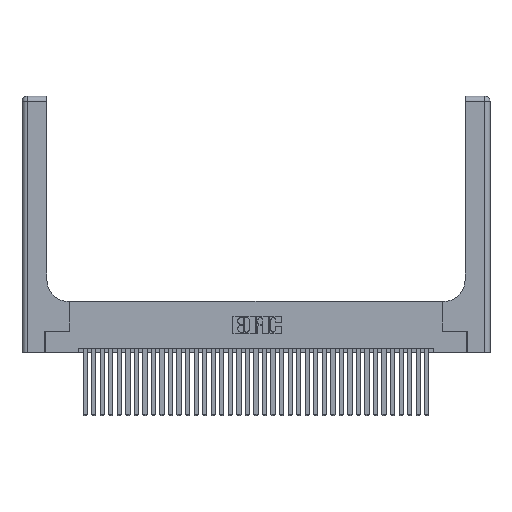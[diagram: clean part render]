
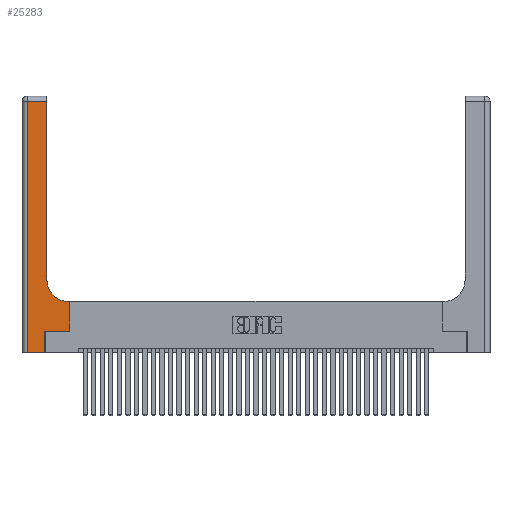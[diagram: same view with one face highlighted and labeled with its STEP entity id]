
A CAD part, top view. The second image highlights one B-rep face of the part: STEP entity #25283.
In plain terms, the highlighted planar face has unit normal (0, 0, 1).
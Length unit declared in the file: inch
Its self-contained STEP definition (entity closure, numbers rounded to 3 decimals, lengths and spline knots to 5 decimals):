
#133 = EDGE_CURVE ( 'NONE', #375, #35585, #22132, .T. ) ;
#169 = CARTESIAN_POINT ( 'NONE',  ( 0.2915, 0.85, 0.37 ) ) ;
#375 = VERTEX_POINT ( 'NONE', #8185 ) ;
#433 = CARTESIAN_POINT ( 'NONE',  ( 0.2915, 0.6, 0.37 ) ) ;
#2279 = CARTESIAN_POINT ( 'NONE',  ( 0., 0., 0.37 ) ) ;
#2367 = VERTEX_POINT ( 'NONE', #33374 ) ;
#2810 = CARTESIAN_POINT ( 'NONE',  ( 0.269, 0., 0.37 ) ) ;
#2972 = LINE ( 'NONE', #32370, #5207 ) ;
#3324 = DIRECTION ( 'NONE',  ( -1., 0., 0. ) ) ;
#3924 = ORIENTED_EDGE ( 'NONE', *, *, #8489, .T. ) ;
#4357 = DIRECTION ( 'NONE',  ( 0., 0., -1. ) ) ;
#4553 = CIRCLE ( 'NONE', #20147, 0.25 ) ;
#4710 = ORIENTED_EDGE ( 'NONE', *, *, #17619, .T. ) ;
#5165 = ORIENTED_EDGE ( 'NONE', *, *, #10488, .T. ) ;
#5207 = VECTOR ( 'NONE', #9206, 39.37008 ) ;
#5732 = DIRECTION ( 'NONE',  ( 0., 0., -1. ) ) ;
#6192 = DIRECTION ( 'NONE',  ( 1., 0., 0. ) ) ;
#6663 = LINE ( 'NONE', #10817, #24252 ) ;
#6765 = CARTESIAN_POINT ( 'NONE',  ( 0., 3., 0.37 ) ) ;
#6771 = ORIENTED_EDGE ( 'NONE', *, *, #24506, .T. ) ;
#7821 = CARTESIAN_POINT ( 'NONE',  ( 0.5585, 0.6, 0.37 ) ) ;
#7998 = VERTEX_POINT ( 'NONE', #28380 ) ;
#8185 = CARTESIAN_POINT ( 'NONE',  ( 0.269, 0.25, 0.37 ) ) ;
#8489 = EDGE_CURVE ( 'NONE', #10835, #26800, #4553, .T. ) ;
#9206 = DIRECTION ( 'NONE',  ( 0., -1., 0. ) ) ;
#9904 = DIRECTION ( 'NONE',  ( -1., 0., 0. ) ) ;
#9983 = EDGE_CURVE ( 'NONE', #24562, #375, #26027, .T. ) ;
#10488 = EDGE_CURVE ( 'NONE', #26800, #16979, #36870, .T. ) ;
#10817 = CARTESIAN_POINT ( 'NONE',  ( 0.5585, 0.25, 0.37 ) ) ;
#10835 = VERTEX_POINT ( 'NONE', #20693 ) ;
#10934 = VECTOR ( 'NONE', #3324, 39.37008 ) ;
#11397 = CARTESIAN_POINT ( 'NONE',  ( 0.269, 0.25, 0.37 ) ) ;
#11854 = ORIENTED_EDGE ( 'NONE', *, *, #18250, .T. ) ;
#12139 = CARTESIAN_POINT ( 'NONE',  ( 0., 2.94, 0.37 ) ) ;
#12611 = VECTOR ( 'NONE', #33770, 39.37008 ) ;
#13055 = LINE ( 'NONE', #2279, #12611 ) ;
#14489 = VECTOR ( 'NONE', #6192, 39.37008 ) ;
#15011 = CARTESIAN_POINT ( 'NONE',  ( 0.269, 0., 0.37 ) ) ;
#15434 = EDGE_LOOP ( 'NONE', ( #5165, #24253, #6771, #4710, #36358, #35288, #11854, #23100, #3924 ) ) ;
#15530 = CARTESIAN_POINT ( 'NONE',  ( 0.5585, 0.25, 0.37 ) ) ;
#15990 = CARTESIAN_POINT ( 'NONE',  ( 0.2915, 3., 0.37 ) ) ;
#16356 = LINE ( 'NONE', #433, #10934 ) ;
#16979 = VERTEX_POINT ( 'NONE', #25038 ) ;
#17619 = EDGE_CURVE ( 'NONE', #2367, #24562, #13055, .T. ) ;
#18250 = EDGE_CURVE ( 'NONE', #35585, #20928, #6663, .T. ) ;
#18481 = PLANE ( 'NONE',  #19754 ) ;
#19015 = DIRECTION ( 'NONE',  ( 0., 1., 0. ) ) ;
#19754 = AXIS2_PLACEMENT_3D ( 'NONE', #6765, #4357, #9904 ) ;
#20147 = AXIS2_PLACEMENT_3D ( 'NONE', #36974, #5732, #31303 ) ;
#20693 = CARTESIAN_POINT ( 'NONE',  ( 0.5415, 0.6, 0.37 ) ) ;
#20928 = VERTEX_POINT ( 'NONE', #7821 ) ;
#21982 = DIRECTION ( 'NONE',  ( 0., 1., 0. ) ) ;
#22132 = LINE ( 'NONE', #11397, #14489 ) ;
#23100 = ORIENTED_EDGE ( 'NONE', *, *, #30639, .T. ) ;
#23702 = DIRECTION ( 'NONE',  ( -1., 0., 0. ) ) ;
#24252 = VECTOR ( 'NONE', #31220, 39.37008 ) ;
#24253 = ORIENTED_EDGE ( 'NONE', *, *, #26421, .T. ) ;
#24506 = EDGE_CURVE ( 'NONE', #7998, #2367, #2972, .T. ) ;
#24562 = VERTEX_POINT ( 'NONE', #15011 ) ;
#24723 = VECTOR ( 'NONE', #19015, 39.37008 ) ;
#25038 = CARTESIAN_POINT ( 'NONE',  ( 0.2915, 2.94, 0.37 ) ) ;
#25283 = ADVANCED_FACE ( 'NONE', ( #32657 ), #18481, .F. ) ;
#26027 = LINE ( 'NONE', #2810, #28808 ) ;
#26421 = EDGE_CURVE ( 'NONE', #16979, #7998, #29500, .T. ) ;
#26800 = VERTEX_POINT ( 'NONE', #169 ) ;
#28380 = CARTESIAN_POINT ( 'NONE',  ( 0.06, 2.94, 0.37 ) ) ;
#28808 = VECTOR ( 'NONE', #21982, 39.37008 ) ;
#29500 = LINE ( 'NONE', #12139, #36239 ) ;
#30639 = EDGE_CURVE ( 'NONE', #20928, #10835, #16356, .T. ) ;
#31220 = DIRECTION ( 'NONE',  ( 0., 1., 0. ) ) ;
#31303 = DIRECTION ( 'NONE',  ( 1., 0., 0. ) ) ;
#32370 = CARTESIAN_POINT ( 'NONE',  ( 0.06, 3., 0.37 ) ) ;
#32657 = FACE_OUTER_BOUND ( 'NONE', #15434, .T. ) ;
#33374 = CARTESIAN_POINT ( 'NONE',  ( 0.06, 0., 0.37 ) ) ;
#33770 = DIRECTION ( 'NONE',  ( 1., 0., 0. ) ) ;
#35288 = ORIENTED_EDGE ( 'NONE', *, *, #133, .T. ) ;
#35585 = VERTEX_POINT ( 'NONE', #15530 ) ;
#36239 = VECTOR ( 'NONE', #23702, 39.37008 ) ;
#36358 = ORIENTED_EDGE ( 'NONE', *, *, #9983, .T. ) ;
#36870 = LINE ( 'NONE', #15990, #24723 ) ;
#36974 = CARTESIAN_POINT ( 'NONE',  ( 0.5415, 0.85, 0.37 ) ) ;
